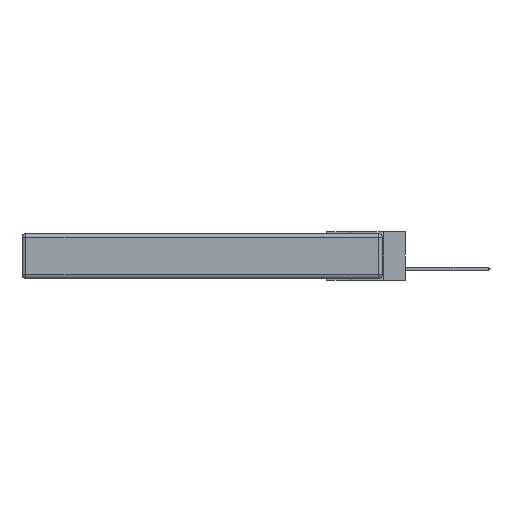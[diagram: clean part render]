
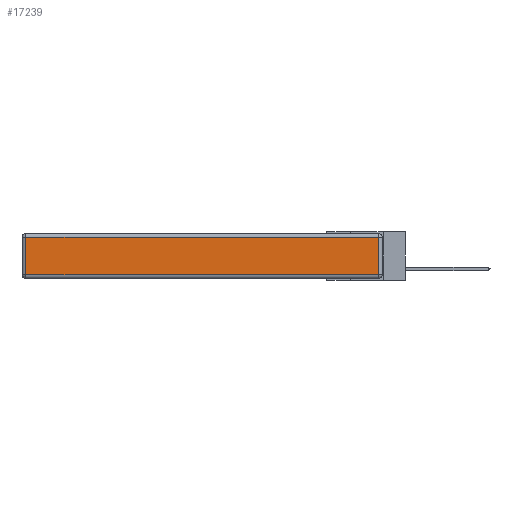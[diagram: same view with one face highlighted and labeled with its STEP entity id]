
A CAD part, left-side view. The second image highlights one B-rep face of the part: STEP entity #17239.
In plain terms, the highlighted planar face has unit normal (-1, 0, 0).
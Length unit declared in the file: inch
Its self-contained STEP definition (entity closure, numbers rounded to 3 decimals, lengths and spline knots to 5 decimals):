
#412 = VERTEX_POINT ( 'NONE', #16669 ) ;
#443 = LINE ( 'NONE', #7232, #17805 ) ;
#475 = DIRECTION ( 'NONE',  ( 0., -1., 0. ) ) ;
#800 = EDGE_CURVE ( 'NONE', #412, #4956, #13081, .T. ) ;
#2709 = DIRECTION ( 'NONE',  ( 0., 0., 1. ) ) ;
#2917 = CARTESIAN_POINT ( 'NONE',  ( 0., 2.72, -0.03 ) ) ;
#3143 = PLANE ( 'NONE',  #8589 ) ;
#4638 = ORIENTED_EDGE ( 'NONE', *, *, #19386, .T. ) ;
#4956 = VERTEX_POINT ( 'NONE', #5388 ) ;
#5220 = VERTEX_POINT ( 'NONE', #18642 ) ;
#5388 = CARTESIAN_POINT ( 'NONE',  ( 0., 0.03, -0.313 ) ) ;
#6850 = DIRECTION ( 'NONE',  ( 0., 0., -1. ) ) ;
#6907 = DIRECTION ( 'NONE',  ( 0., 1., 0. ) ) ;
#7232 = CARTESIAN_POINT ( 'NONE',  ( 0., 0.03, -0.343 ) ) ;
#7523 = FACE_OUTER_BOUND ( 'NONE', #11284, .T. ) ;
#8489 = ORIENTED_EDGE ( 'NONE', *, *, #13466, .T. ) ;
#8589 = AXIS2_PLACEMENT_3D ( 'NONE', #13748, #15253, #13611 ) ;
#9638 = ORIENTED_EDGE ( 'NONE', *, *, #800, .T. ) ;
#10521 = LINE ( 'NONE', #11316, #17378 ) ;
#11284 = EDGE_LOOP ( 'NONE', ( #9638, #19201, #8489, #4638 ) ) ;
#11316 = CARTESIAN_POINT ( 'NONE',  ( 0., 2.75, -0.03 ) ) ;
#12730 = CARTESIAN_POINT ( 'NONE',  ( 0., 0., -0.313 ) ) ;
#13081 = LINE ( 'NONE', #12730, #13527 ) ;
#13466 = EDGE_CURVE ( 'NONE', #5220, #17049, #10521, .T. ) ;
#13527 = VECTOR ( 'NONE', #475, 39.37008 ) ;
#13611 = DIRECTION ( 'NONE',  ( 0., 0., 1. ) ) ;
#13748 = CARTESIAN_POINT ( 'NONE',  ( 0., 0., -0.343 ) ) ;
#14881 = LINE ( 'NONE', #17107, #18197 ) ;
#15253 = DIRECTION ( 'NONE',  ( -1., 0., 0. ) ) ;
#16669 = CARTESIAN_POINT ( 'NONE',  ( 0., 2.72, -0.313 ) ) ;
#17049 = VERTEX_POINT ( 'NONE', #2917 ) ;
#17107 = CARTESIAN_POINT ( 'NONE',  ( 0., 2.72, -0.343 ) ) ;
#17239 = ADVANCED_FACE ( 'NONE', ( #7523 ), #3143, .T. ) ;
#17378 = VECTOR ( 'NONE', #6907, 39.37008 ) ;
#17759 = EDGE_CURVE ( 'NONE', #4956, #5220, #443, .T. ) ;
#17805 = VECTOR ( 'NONE', #2709, 39.37008 ) ;
#18197 = VECTOR ( 'NONE', #6850, 39.37008 ) ;
#18642 = CARTESIAN_POINT ( 'NONE',  ( 0., 0.03, -0.03 ) ) ;
#19201 = ORIENTED_EDGE ( 'NONE', *, *, #17759, .T. ) ;
#19386 = EDGE_CURVE ( 'NONE', #17049, #412, #14881, .T. ) ;
